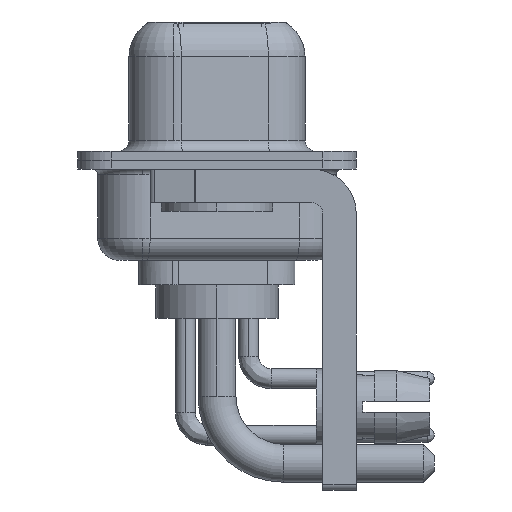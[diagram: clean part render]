
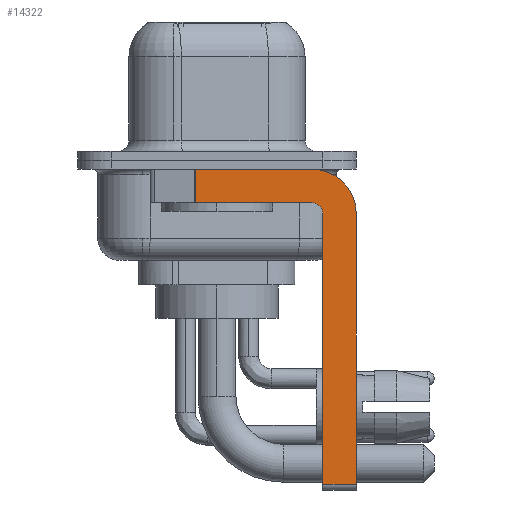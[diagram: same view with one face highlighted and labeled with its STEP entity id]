
A CAD part, left-side view. The second image highlights one B-rep face of the part: STEP entity #14322.
In plain terms, the highlighted planar face has unit normal (-1, 0, 0).
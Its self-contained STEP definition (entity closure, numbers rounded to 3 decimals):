
#720 = CARTESIAN_POINT ( 'NONE',  ( -2.9, -6.25, -14.55 ) ) ;
#892 = CARTESIAN_POINT ( 'NONE',  ( -2.9, -4.25, -2.4 ) ) ;
#924 = ORIENTED_EDGE ( 'NONE', *, *, #15396, .F. ) ;
#925 = VECTOR ( 'NONE', #6376, 1000. ) ;
#1377 = PLANE ( 'NONE',  #10356 ) ;
#1974 = DIRECTION ( 'NONE',  ( 1., 0., 0. ) ) ;
#2031 = VECTOR ( 'NONE', #19904, 1000. ) ;
#2171 = ORIENTED_EDGE ( 'NONE', *, *, #10584, .T. ) ;
#2624 = CARTESIAN_POINT ( 'NONE',  ( -2.9, -4.25, -2.4 ) ) ;
#2958 = EDGE_CURVE ( 'NONE', #11488, #9121, #12732, .T. ) ;
#3178 = AXIS2_PLACEMENT_3D ( 'NONE', #2624, #22044, #5946 ) ;
#3601 = CIRCLE ( 'NONE', #6624, 0.5 ) ;
#4513 = CARTESIAN_POINT ( 'NONE',  ( -2.9, 3., -0.4 ) ) ;
#4539 = DIRECTION ( 'NONE',  ( -1., 0., 0. ) ) ;
#4600 = ORIENTED_EDGE ( 'NONE', *, *, #15848, .F. ) ;
#5171 = CARTESIAN_POINT ( 'NONE',  ( -2.9, -6.25, -2.4 ) ) ;
#5249 = VERTEX_POINT ( 'NONE', #21547 ) ;
#5257 = CARTESIAN_POINT ( 'NONE',  ( -2.9, -4.25, -14.55 ) ) ;
#5425 = VECTOR ( 'NONE', #6287, 1000. ) ;
#5624 = VERTEX_POINT ( 'NONE', #19818 ) ;
#5946 = DIRECTION ( 'NONE',  ( 0., 0., -1. ) ) ;
#6287 = DIRECTION ( 'NONE',  ( 0., -1., 0. ) ) ;
#6376 = DIRECTION ( 'NONE',  ( 0., 1., 0. ) ) ;
#6624 = AXIS2_PLACEMENT_3D ( 'NONE', #892, #4539, #22415 ) ;
#7027 = ORIENTED_EDGE ( 'NONE', *, *, #8476, .F. ) ;
#7095 = VERTEX_POINT ( 'NONE', #16209 ) ;
#7416 = ORIENTED_EDGE ( 'NONE', *, *, #9431, .F. ) ;
#8085 = CARTESIAN_POINT ( 'NONE',  ( -2.9, -4.75, -2.4 ) ) ;
#8476 = EDGE_CURVE ( 'NONE', #5624, #10178, #16657, .T. ) ;
#9121 = VERTEX_POINT ( 'NONE', #14264 ) ;
#9431 = EDGE_CURVE ( 'NONE', #7095, #19132, #10248, .T. ) ;
#10178 = VERTEX_POINT ( 'NONE', #8085 ) ;
#10248 = LINE ( 'NONE', #5171, #17702 ) ;
#10356 = AXIS2_PLACEMENT_3D ( 'NONE', #18180, #1974, #10573 ) ;
#10398 = ORIENTED_EDGE ( 'NONE', *, *, #2958, .T. ) ;
#10573 = DIRECTION ( 'NONE',  ( 0., 0., -1. ) ) ;
#10584 = EDGE_CURVE ( 'NONE', #5624, #19132, #14563, .T. ) ;
#11488 = VERTEX_POINT ( 'NONE', #18452 ) ;
#11881 = VERTEX_POINT ( 'NONE', #20814 ) ;
#11902 = ORIENTED_EDGE ( 'NONE', *, *, #17728, .F. ) ;
#12087 = FACE_OUTER_BOUND ( 'NONE', #12762, .T. ) ;
#12732 = LINE ( 'NONE', #20143, #2031 ) ;
#12762 = EDGE_LOOP ( 'NONE', ( #17589, #10398, #11902, #924, #7027, #2171, #7416, #4600 ) ) ;
#14264 = CARTESIAN_POINT ( 'NONE',  ( -2.9, 0.978, -1.9 ) ) ;
#14322 = ADVANCED_FACE ( 'NONE', ( #12087 ), #1377, .F. ) ;
#14563 = LINE ( 'NONE', #5257, #20394 ) ;
#14917 = DIRECTION ( 'NONE',  ( 0., 0., 1. ) ) ;
#15396 = EDGE_CURVE ( 'NONE', #10178, #11881, #3601, .T. ) ;
#15656 = CARTESIAN_POINT ( 'NONE',  ( -2.9, -4.25, -1.9 ) ) ;
#15848 = EDGE_CURVE ( 'NONE', #5249, #7095, #20076, .T. ) ;
#16209 = CARTESIAN_POINT ( 'NONE',  ( -2.9, -6.25, -2.4 ) ) ;
#16632 = LINE ( 'NONE', #4513, #5425 ) ;
#16657 = LINE ( 'NONE', #16767, #20312 ) ;
#16767 = CARTESIAN_POINT ( 'NONE',  ( -2.9, -4.75, -14.8 ) ) ;
#17079 = EDGE_CURVE ( 'NONE', #11488, #5249, #16632, .T. ) ;
#17589 = ORIENTED_EDGE ( 'NONE', *, *, #17079, .F. ) ;
#17617 = DIRECTION ( 'NONE',  ( 0., 0., -1. ) ) ;
#17702 = VECTOR ( 'NONE', #17617, 1000. ) ;
#17728 = EDGE_CURVE ( 'NONE', #11881, #9121, #19279, .T. ) ;
#18053 = DIRECTION ( 'NONE',  ( 0., -1., 0. ) ) ;
#18180 = CARTESIAN_POINT ( 'NONE',  ( -2.9, -4.25, -2.4 ) ) ;
#18452 = CARTESIAN_POINT ( 'NONE',  ( -2.9, 0.978, -0.4 ) ) ;
#19132 = VERTEX_POINT ( 'NONE', #720 ) ;
#19279 = LINE ( 'NONE', #15656, #925 ) ;
#19818 = CARTESIAN_POINT ( 'NONE',  ( -2.9, -4.75, -14.55 ) ) ;
#19904 = DIRECTION ( 'NONE',  ( 0., 0., -1. ) ) ;
#20076 = CIRCLE ( 'NONE', #3178, 2. ) ;
#20143 = CARTESIAN_POINT ( 'NONE',  ( -2.9, 0.978, -1.9 ) ) ;
#20312 = VECTOR ( 'NONE', #14917, 1000. ) ;
#20394 = VECTOR ( 'NONE', #18053, 1000. ) ;
#20814 = CARTESIAN_POINT ( 'NONE',  ( -2.9, -4.25, -1.9 ) ) ;
#21547 = CARTESIAN_POINT ( 'NONE',  ( -2.9, -4.25, -0.4 ) ) ;
#22044 = DIRECTION ( 'NONE',  ( 1., 0., 0. ) ) ;
#22415 = DIRECTION ( 'NONE',  ( 0., 0., 1. ) ) ;
